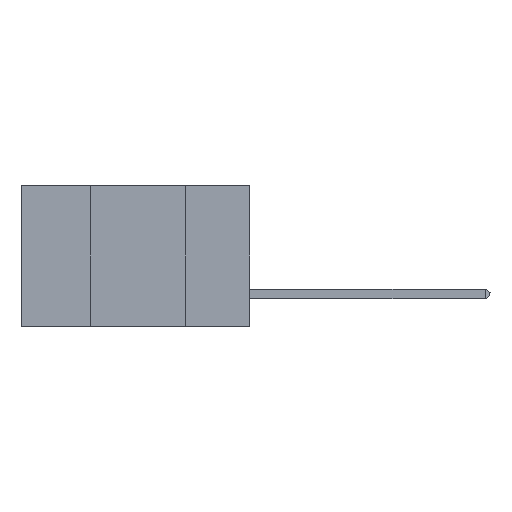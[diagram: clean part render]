
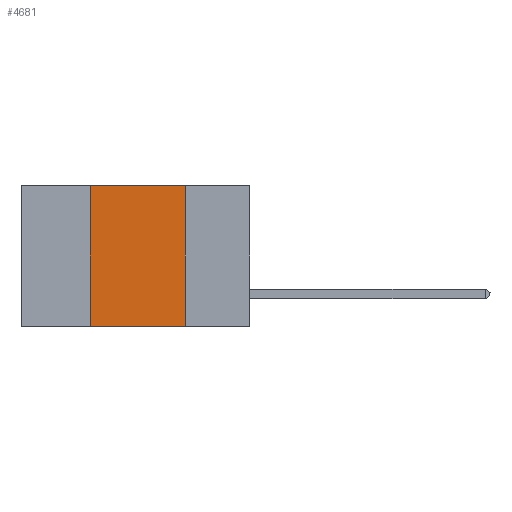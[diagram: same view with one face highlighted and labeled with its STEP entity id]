
A CAD part, left-side view. The second image highlights one B-rep face of the part: STEP entity #4681.
In plain terms, the highlighted planar face has unit normal (-1, 0, 0).
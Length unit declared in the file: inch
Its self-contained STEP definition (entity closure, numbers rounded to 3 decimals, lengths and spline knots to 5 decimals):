
#535 = VECTOR ( 'NONE', #4143, 39.37008 ) ;
#956 = VERTEX_POINT ( 'NONE', #31881 ) ;
#1024 = ORIENTED_EDGE ( 'NONE', *, *, #14622, .T. ) ;
#1540 = LINE ( 'NONE', #17342, #13506 ) ;
#2400 = CARTESIAN_POINT ( 'NONE',  ( 0., 0.6, -0.37 ) ) ;
#3448 = PLANE ( 'NONE',  #22497 ) ;
#4143 = DIRECTION ( 'NONE',  ( 0., 0., -1. ) ) ;
#4681 = ADVANCED_FACE ( 'NONE', ( #15475 ), #3448, .F. ) ;
#6221 = CARTESIAN_POINT ( 'NONE',  ( 0., 0.6, 0. ) ) ;
#6663 = CARTESIAN_POINT ( 'NONE',  ( 0., 0.17, 0. ) ) ;
#6748 = CARTESIAN_POINT ( 'NONE',  ( 0., 0.42, 0. ) ) ;
#6922 = VECTOR ( 'NONE', #21438, 39.37008 ) ;
#8944 = DIRECTION ( 'NONE',  ( 0., 0., -1. ) ) ;
#10386 = VERTEX_POINT ( 'NONE', #35391 ) ;
#12619 = VERTEX_POINT ( 'NONE', #22504 ) ;
#12711 = EDGE_CURVE ( 'NONE', #12619, #956, #22310, .T. ) ;
#12872 = LINE ( 'NONE', #2400, #6922 ) ;
#13506 = VECTOR ( 'NONE', #22730, 39.37008 ) ;
#14622 = EDGE_CURVE ( 'NONE', #10386, #956, #12872, .T. ) ;
#14659 = ORIENTED_EDGE ( 'NONE', *, *, #28262, .F. ) ;
#15475 = FACE_OUTER_BOUND ( 'NONE', #34289, .T. ) ;
#15698 = ORIENTED_EDGE ( 'NONE', *, *, #18524, .F. ) ;
#17342 = CARTESIAN_POINT ( 'NONE',  ( 0., 0.42, 0. ) ) ;
#18006 = CARTESIAN_POINT ( 'NONE',  ( 0., 0.6, 0. ) ) ;
#18524 = EDGE_CURVE ( 'NONE', #23092, #12619, #30929, .T. ) ;
#21438 = DIRECTION ( 'NONE',  ( 0., -1., 0. ) ) ;
#22310 = LINE ( 'NONE', #6663, #535 ) ;
#22497 = AXIS2_PLACEMENT_3D ( 'NONE', #6221, #25289, #8944 ) ;
#22504 = CARTESIAN_POINT ( 'NONE',  ( 0., 0.17, 0. ) ) ;
#22730 = DIRECTION ( 'NONE',  ( 0., 0., 1. ) ) ;
#23092 = VERTEX_POINT ( 'NONE', #6748 ) ;
#25289 = DIRECTION ( 'NONE',  ( 1., 0., 0. ) ) ;
#26342 = ORIENTED_EDGE ( 'NONE', *, *, #12711, .F. ) ;
#28262 = EDGE_CURVE ( 'NONE', #10386, #23092, #1540, .T. ) ;
#28643 = DIRECTION ( 'NONE',  ( 0., -1., 0. ) ) ;
#30049 = VECTOR ( 'NONE', #28643, 39.37008 ) ;
#30929 = LINE ( 'NONE', #18006, #30049 ) ;
#31881 = CARTESIAN_POINT ( 'NONE',  ( 0., 0.17, -0.37 ) ) ;
#34289 = EDGE_LOOP ( 'NONE', ( #26342, #15698, #14659, #1024 ) ) ;
#35391 = CARTESIAN_POINT ( 'NONE',  ( 0., 0.42, -0.37 ) ) ;
